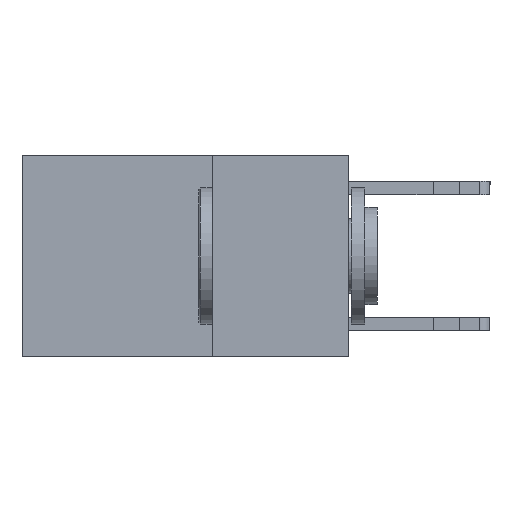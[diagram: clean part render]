
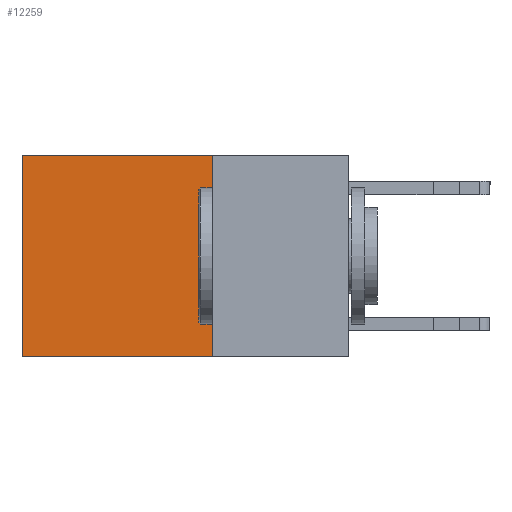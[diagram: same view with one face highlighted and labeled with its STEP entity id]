
A CAD part, left-side view. The second image highlights one B-rep face of the part: STEP entity #12259.
In plain terms, the highlighted planar face has unit normal (-1, 0, 0).
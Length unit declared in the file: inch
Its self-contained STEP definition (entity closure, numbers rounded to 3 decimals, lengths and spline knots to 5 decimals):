
#628 = EDGE_CURVE ( 'NONE', #15143, #3318, #4583, .T. ) ;
#1939 = DIRECTION ( 'NONE',  ( 1., 0., 0. ) ) ;
#2077 = FACE_OUTER_BOUND ( 'NONE', #3067, .T. ) ;
#2257 = VECTOR ( 'NONE', #11119, 39.37008 ) ;
#2517 = CARTESIAN_POINT ( 'NONE',  ( 0.2625, 0.6, 0. ) ) ;
#2885 = CARTESIAN_POINT ( 'NONE',  ( 0.2625, 0.25, -0.37 ) ) ;
#3067 = EDGE_LOOP ( 'NONE', ( #26205, #21629, #24962, #24711 ) ) ;
#3318 = VERTEX_POINT ( 'NONE', #21945 ) ;
#4583 = LINE ( 'NONE', #17841, #11450 ) ;
#5321 = DIRECTION ( 'NONE',  ( 0., 1., 0. ) ) ;
#6296 = PLANE ( 'NONE',  #10255 ) ;
#7767 = VECTOR ( 'NONE', #5321, 39.37008 ) ;
#9510 = CARTESIAN_POINT ( 'NONE',  ( 0.2625, 0.6, -0.37 ) ) ;
#10255 = AXIS2_PLACEMENT_3D ( 'NONE', #12310, #1939, #18354 ) ;
#10914 = VERTEX_POINT ( 'NONE', #16429 ) ;
#11119 = DIRECTION ( 'NONE',  ( 0., 0., -1. ) ) ;
#11450 = VECTOR ( 'NONE', #26416, 39.37008 ) ;
#12259 = ADVANCED_FACE ( 'NONE', ( #2077 ), #6296, .F. ) ;
#12310 = CARTESIAN_POINT ( 'NONE',  ( 0.2625, 0.25, 0. ) ) ;
#13529 = DIRECTION ( 'NONE',  ( 0., 1., 0. ) ) ;
#15143 = VERTEX_POINT ( 'NONE', #20884 ) ;
#16429 = CARTESIAN_POINT ( 'NONE',  ( 0.2625, 0.6, 0. ) ) ;
#16757 = VERTEX_POINT ( 'NONE', #9510 ) ;
#16971 = VECTOR ( 'NONE', #13529, 39.37008 ) ;
#17375 = EDGE_CURVE ( 'NONE', #15143, #10914, #17918, .T. ) ;
#17653 = EDGE_CURVE ( 'NONE', #3318, #16757, #23638, .T. ) ;
#17841 = CARTESIAN_POINT ( 'NONE',  ( 0.2625, 0.25, 0. ) ) ;
#17918 = LINE ( 'NONE', #21973, #7767 ) ;
#18354 = DIRECTION ( 'NONE',  ( 0., 0., -1. ) ) ;
#20514 = EDGE_CURVE ( 'NONE', #10914, #16757, #25741, .T. ) ;
#20884 = CARTESIAN_POINT ( 'NONE',  ( 0.2625, 0.25, 0. ) ) ;
#21629 = ORIENTED_EDGE ( 'NONE', *, *, #17653, .F. ) ;
#21945 = CARTESIAN_POINT ( 'NONE',  ( 0.2625, 0.25, -0.37 ) ) ;
#21973 = CARTESIAN_POINT ( 'NONE',  ( 0.2625, 0.25, 0. ) ) ;
#23638 = LINE ( 'NONE', #2885, #16971 ) ;
#24711 = ORIENTED_EDGE ( 'NONE', *, *, #17375, .T. ) ;
#24962 = ORIENTED_EDGE ( 'NONE', *, *, #628, .F. ) ;
#25741 = LINE ( 'NONE', #2517, #2257 ) ;
#26205 = ORIENTED_EDGE ( 'NONE', *, *, #20514, .T. ) ;
#26416 = DIRECTION ( 'NONE',  ( 0., 0., -1. ) ) ;
